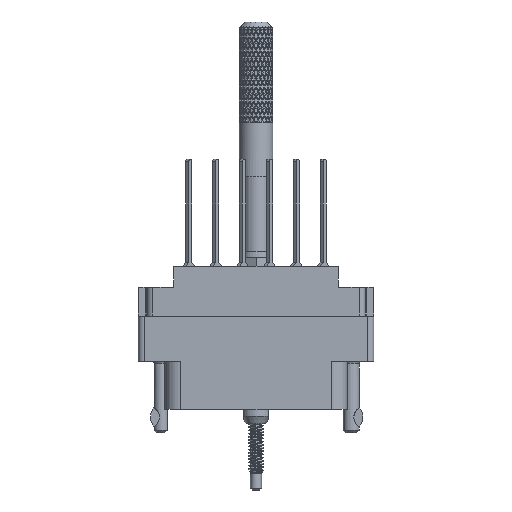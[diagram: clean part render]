
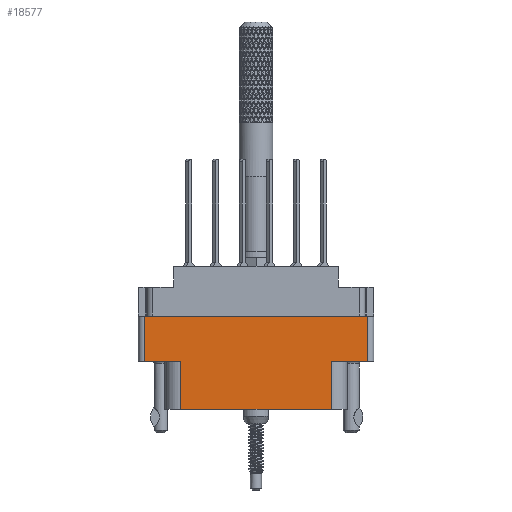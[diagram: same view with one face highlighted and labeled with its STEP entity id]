
A CAD part, front view. The second image highlights one B-rep face of the part: STEP entity #18577.
In plain terms, the highlighted planar face has unit normal (0, -1, 0).
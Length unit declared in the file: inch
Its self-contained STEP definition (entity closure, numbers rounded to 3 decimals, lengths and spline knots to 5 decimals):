
#1731 = DIRECTION ( 'NONE',  ( 0., 0., -1. ) ) ;
#4846 = CARTESIAN_POINT ( 'NONE',  ( -0.624, -0.343, -0.798 ) ) ;
#9204 = LINE ( 'NONE', #4846, #155850 ) ;
#10919 = ORIENTED_EDGE ( 'NONE', *, *, #85949, .F. ) ;
#14469 = VERTEX_POINT ( 'NONE', #168424 ) ;
#18577 = ADVANCED_FACE ( 'NONE', ( #51271 ), #109871, .T. ) ;
#19564 = DIRECTION ( 'NONE',  ( 0., 0., -1. ) ) ;
#19730 = DIRECTION ( 'NONE',  ( -1., 0., 0. ) ) ;
#19977 = EDGE_CURVE ( 'NONE', #14469, #89552, #50906, .T. ) ;
#24439 = VECTOR ( 'NONE', #19730, 39.37008 ) ;
#29046 = VECTOR ( 'NONE', #152767, 39.37008 ) ;
#33283 = ORIENTED_EDGE ( 'NONE', *, *, #189131, .F. ) ;
#34318 = VERTEX_POINT ( 'NONE', #153072 ) ;
#41005 = ORIENTED_EDGE ( 'NONE', *, *, #81304, .T. ) ;
#47851 = EDGE_CURVE ( 'NONE', #106764, #117896, #62526, .T. ) ;
#50613 = CARTESIAN_POINT ( 'NONE',  ( -0.624, -0.343, -0.798 ) ) ;
#50906 = LINE ( 'NONE', #77653, #139534 ) ;
#51271 = FACE_OUTER_BOUND ( 'NONE', #186879, .T. ) ;
#56589 = VERTEX_POINT ( 'NONE', #69975 ) ;
#62526 = LINE ( 'NONE', #139041, #153359 ) ;
#69975 = CARTESIAN_POINT ( 'NONE',  ( 0.42, -0.343, -0.529 ) ) ;
#71074 = CARTESIAN_POINT ( 'NONE',  ( 0.624, -0.343, -0.529 ) ) ;
#77653 = CARTESIAN_POINT ( 'NONE',  ( -0.624, -0.343, -0.798 ) ) ;
#79664 = CARTESIAN_POINT ( 'NONE',  ( 0., -0.343, -0.529 ) ) ;
#80624 = DIRECTION ( 'NONE',  ( 0., -1., 0. ) ) ;
#80765 = VECTOR ( 'NONE', #1731, 39.37008 ) ;
#80817 = LINE ( 'NONE', #88915, #162271 ) ;
#81304 = EDGE_CURVE ( 'NONE', #172043, #34318, #80817, .T. ) ;
#83087 = AXIS2_PLACEMENT_3D ( 'NONE', #50613, #80624, #112454 ) ;
#85949 = EDGE_CURVE ( 'NONE', #172043, #56589, #161937, .T. ) ;
#88915 = CARTESIAN_POINT ( 'NONE',  ( 0.624, -0.343, -0.798 ) ) ;
#89552 = VERTEX_POINT ( 'NONE', #165425 ) ;
#90537 = EDGE_CURVE ( 'NONE', #56589, #89552, #181543, .T. ) ;
#91174 = ORIENTED_EDGE ( 'NONE', *, *, #19977, .T. ) ;
#92035 = ORIENTED_EDGE ( 'NONE', *, *, #166128, .F. ) ;
#93485 = DIRECTION ( 'NONE',  ( 1., 0., 0. ) ) ;
#94607 = DIRECTION ( 'NONE',  ( 0., 0., 1. ) ) ;
#100132 = ORIENTED_EDGE ( 'NONE', *, *, #180248, .T. ) ;
#106764 = VERTEX_POINT ( 'NONE', #151438 ) ;
#109871 = PLANE ( 'NONE',  #83087 ) ;
#112454 = DIRECTION ( 'NONE',  ( 0., 0., -1. ) ) ;
#114722 = CARTESIAN_POINT ( 'NONE',  ( -0.624, -0.343, -0.277 ) ) ;
#115597 = LINE ( 'NONE', #139106, #80765 ) ;
#117896 = VERTEX_POINT ( 'NONE', #129897 ) ;
#119446 = DIRECTION ( 'NONE',  ( 0., 0., 1. ) ) ;
#119521 = CARTESIAN_POINT ( 'NONE',  ( -0.656, -0.343, -0.277 ) ) ;
#129772 = VERTEX_POINT ( 'NONE', #114722 ) ;
#129897 = CARTESIAN_POINT ( 'NONE',  ( -0.42, -0.343, -0.529 ) ) ;
#139041 = CARTESIAN_POINT ( 'NONE',  ( 0., -0.343, -0.529 ) ) ;
#139106 = CARTESIAN_POINT ( 'NONE',  ( -0.42, -0.343, -0.529 ) ) ;
#139534 = VECTOR ( 'NONE', #167578, 39.37008 ) ;
#147993 = LINE ( 'NONE', #119521, #29046 ) ;
#149884 = CARTESIAN_POINT ( 'NONE',  ( 0.42, -0.343, -0.529 ) ) ;
#151438 = CARTESIAN_POINT ( 'NONE',  ( -0.624, -0.343, -0.529 ) ) ;
#152767 = DIRECTION ( 'NONE',  ( 1., 0., 0. ) ) ;
#153072 = CARTESIAN_POINT ( 'NONE',  ( 0.624, -0.343, -0.277 ) ) ;
#153359 = VECTOR ( 'NONE', #93485, 39.37008 ) ;
#155850 = VECTOR ( 'NONE', #94607, 39.37008 ) ;
#161937 = LINE ( 'NONE', #79664, #24439 ) ;
#162271 = VECTOR ( 'NONE', #119446, 39.37008 ) ;
#164626 = ORIENTED_EDGE ( 'NONE', *, *, #47851, .T. ) ;
#165425 = CARTESIAN_POINT ( 'NONE',  ( 0.42, -0.343, -0.798 ) ) ;
#166128 = EDGE_CURVE ( 'NONE', #129772, #34318, #147993, .T. ) ;
#167578 = DIRECTION ( 'NONE',  ( 1., 0., 0. ) ) ;
#168424 = CARTESIAN_POINT ( 'NONE',  ( -0.42, -0.343, -0.798 ) ) ;
#172043 = VERTEX_POINT ( 'NONE', #71074 ) ;
#172196 = VECTOR ( 'NONE', #19564, 39.37008 ) ;
#180248 = EDGE_CURVE ( 'NONE', #117896, #14469, #115597, .T. ) ;
#181543 = LINE ( 'NONE', #149884, #172196 ) ;
#182641 = ORIENTED_EDGE ( 'NONE', *, *, #90537, .F. ) ;
#186879 = EDGE_LOOP ( 'NONE', ( #100132, #91174, #182641, #10919, #41005, #92035, #33283, #164626 ) ) ;
#189131 = EDGE_CURVE ( 'NONE', #106764, #129772, #9204, .T. ) ;
